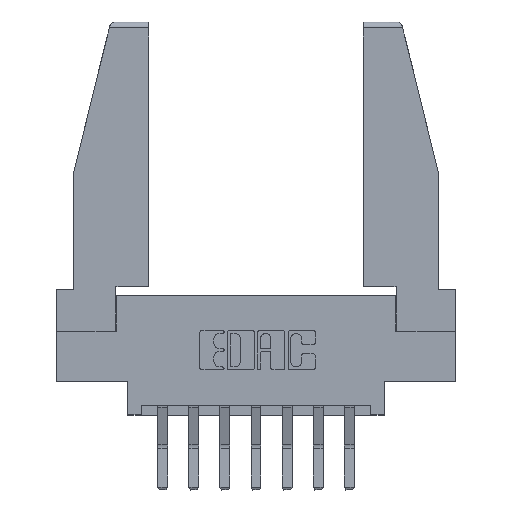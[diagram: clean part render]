
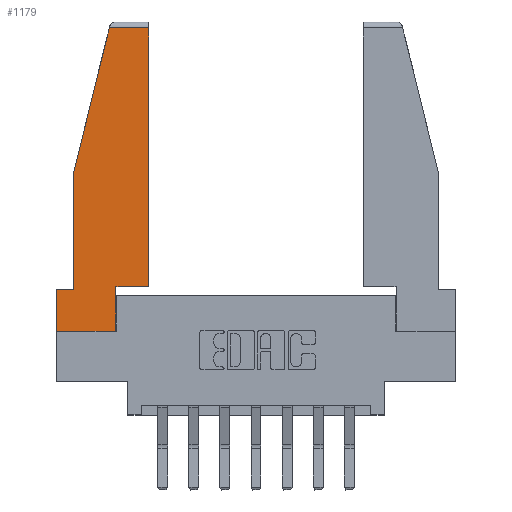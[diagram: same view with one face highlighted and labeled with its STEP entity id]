
A CAD part, top view. The second image highlights one B-rep face of the part: STEP entity #1179.
In plain terms, the highlighted planar face has unit normal (0, 0, 1).
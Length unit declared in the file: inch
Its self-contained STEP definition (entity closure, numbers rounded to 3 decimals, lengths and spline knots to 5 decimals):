
#137 = VERTEX_POINT ( 'NONE', #3178 ) ;
#279 = CARTESIAN_POINT ( 'NONE',  ( 0., 0.21, 0. ) ) ;
#529 = VERTEX_POINT ( 'NONE', #4607 ) ;
#646 = DIRECTION ( 'NONE',  ( 1., 0., 0. ) ) ;
#731 = EDGE_CURVE ( 'NONE', #529, #7442, #9859, .T. ) ;
#817 = PLANE ( 'NONE',  #4646 ) ;
#908 = VERTEX_POINT ( 'NONE', #1582 ) ;
#1040 = VECTOR ( 'NONE', #3634, 39.37008 ) ;
#1179 = ADVANCED_FACE ( 'NONE', ( #3881 ), #817, .T. ) ;
#1341 = LINE ( 'NONE', #5484, #3326 ) ;
#1395 = CARTESIAN_POINT ( 'NONE',  ( 0.086, 0.21, 0. ) ) ;
#1582 = CARTESIAN_POINT ( 'NONE',  ( 0.461, 1.52, 0. ) ) ;
#1801 = DIRECTION ( 'NONE',  ( 0., 0., 1. ) ) ;
#2107 = VERTEX_POINT ( 'NONE', #4416 ) ;
#2171 = DIRECTION ( 'NONE',  ( 1., 0., 0. ) ) ;
#2266 = VERTEX_POINT ( 'NONE', #9432 ) ;
#2428 = CARTESIAN_POINT ( 'NONE',  ( 0., 0., 0. ) ) ;
#2433 = ORIENTED_EDGE ( 'NONE', *, *, #7986, .T. ) ;
#2893 = CARTESIAN_POINT ( 'NONE',  ( 0.271, 1.55, 0. ) ) ;
#3178 = CARTESIAN_POINT ( 'NONE',  ( 0.086, 0.8, 0. ) ) ;
#3216 = CARTESIAN_POINT ( 'NONE',  ( 0.297, 0., 0. ) ) ;
#3251 = VERTEX_POINT ( 'NONE', #12536 ) ;
#3326 = VECTOR ( 'NONE', #646, 39.37008 ) ;
#3634 = DIRECTION ( 'NONE',  ( 0., 1., 0. ) ) ;
#3812 = DIRECTION ( 'NONE',  ( 1., 0., 0. ) ) ;
#3881 = FACE_OUTER_BOUND ( 'NONE', #4019, .T. ) ;
#3917 = DIRECTION ( 'NONE',  ( -0.239, -0.971, 0. ) ) ;
#4019 = EDGE_LOOP ( 'NONE', ( #8978, #4724, #11469, #11731, #11150, #2433, #6313, #5089, #8699 ) ) ;
#4416 = CARTESIAN_POINT ( 'NONE',  ( 0., 0.21, 0. ) ) ;
#4423 = EDGE_CURVE ( 'NONE', #137, #7689, #7881, .T. ) ;
#4431 = CARTESIAN_POINT ( 'NONE',  ( 0.086, 0.8, 0. ) ) ;
#4607 = CARTESIAN_POINT ( 'NONE',  ( 0.297, 0., 0. ) ) ;
#4643 = EDGE_CURVE ( 'NONE', #908, #3251, #8922, .T. ) ;
#4646 = AXIS2_PLACEMENT_3D ( 'NONE', #12539, #1801, #3812 ) ;
#4724 = ORIENTED_EDGE ( 'NONE', *, *, #4643, .T. ) ;
#5028 = VECTOR ( 'NONE', #2171, 39.37008 ) ;
#5089 = ORIENTED_EDGE ( 'NONE', *, *, #731, .T. ) ;
#5275 = VECTOR ( 'NONE', #5289, 39.37008 ) ;
#5289 = DIRECTION ( 'NONE',  ( 0., -1., 0. ) ) ;
#5484 = CARTESIAN_POINT ( 'NONE',  ( 0., 0., 0. ) ) ;
#5758 = CARTESIAN_POINT ( 'NONE',  ( 0.297, 0.223, 0. ) ) ;
#6037 = DIRECTION ( 'NONE',  ( 0., 1., 0. ) ) ;
#6171 = CARTESIAN_POINT ( 'NONE',  ( 0.297, 0.223, 0. ) ) ;
#6313 = ORIENTED_EDGE ( 'NONE', *, *, #9028, .T. ) ;
#6862 = LINE ( 'NONE', #279, #11810 ) ;
#7442 = VERTEX_POINT ( 'NONE', #5758 ) ;
#7689 = VERTEX_POINT ( 'NONE', #1395 ) ;
#7881 = LINE ( 'NONE', #4431, #5275 ) ;
#7986 = EDGE_CURVE ( 'NONE', #2107, #10548, #9282, .T. ) ;
#8084 = CARTESIAN_POINT ( 'NONE',  ( 0., 1.52, 0. ) ) ;
#8699 = ORIENTED_EDGE ( 'NONE', *, *, #9233, .T. ) ;
#8922 = LINE ( 'NONE', #8084, #12156 ) ;
#8978 = ORIENTED_EDGE ( 'NONE', *, *, #9063, .T. ) ;
#9028 = EDGE_CURVE ( 'NONE', #10548, #529, #1341, .T. ) ;
#9063 = EDGE_CURVE ( 'NONE', #2266, #908, #11608, .T. ) ;
#9233 = EDGE_CURVE ( 'NONE', #7442, #2266, #9438, .T. ) ;
#9282 = LINE ( 'NONE', #9861, #11287 ) ;
#9432 = CARTESIAN_POINT ( 'NONE',  ( 0.461, 0.223, 0. ) ) ;
#9438 = LINE ( 'NONE', #6171, #5028 ) ;
#9780 = DIRECTION ( 'NONE',  ( 0., -1., 0. ) ) ;
#9859 = LINE ( 'NONE', #3216, #11550 ) ;
#9861 = CARTESIAN_POINT ( 'NONE',  ( 0., 0.21, 0. ) ) ;
#9956 = DIRECTION ( 'NONE',  ( -1., 0., 0. ) ) ;
#10306 = EDGE_CURVE ( 'NONE', #3251, #137, #12202, .T. ) ;
#10548 = VERTEX_POINT ( 'NONE', #2428 ) ;
#10586 = CARTESIAN_POINT ( 'NONE',  ( 0.461, 0.223, 0. ) ) ;
#11150 = ORIENTED_EDGE ( 'NONE', *, *, #11862, .T. ) ;
#11287 = VECTOR ( 'NONE', #9780, 39.37008 ) ;
#11469 = ORIENTED_EDGE ( 'NONE', *, *, #10306, .T. ) ;
#11550 = VECTOR ( 'NONE', #6037, 39.37008 ) ;
#11608 = LINE ( 'NONE', #10586, #1040 ) ;
#11731 = ORIENTED_EDGE ( 'NONE', *, *, #4423, .T. ) ;
#11810 = VECTOR ( 'NONE', #11909, 39.37008 ) ;
#11862 = EDGE_CURVE ( 'NONE', #7689, #2107, #6862, .T. ) ;
#11902 = VECTOR ( 'NONE', #3917, 39.37008 ) ;
#11909 = DIRECTION ( 'NONE',  ( -1., 0., 0. ) ) ;
#12156 = VECTOR ( 'NONE', #9956, 39.37008 ) ;
#12202 = LINE ( 'NONE', #2893, #11902 ) ;
#12536 = CARTESIAN_POINT ( 'NONE',  ( 0.2636, 1.52, 0. ) ) ;
#12539 = CARTESIAN_POINT ( 'NONE',  ( 0., 0., 0. ) ) ;
